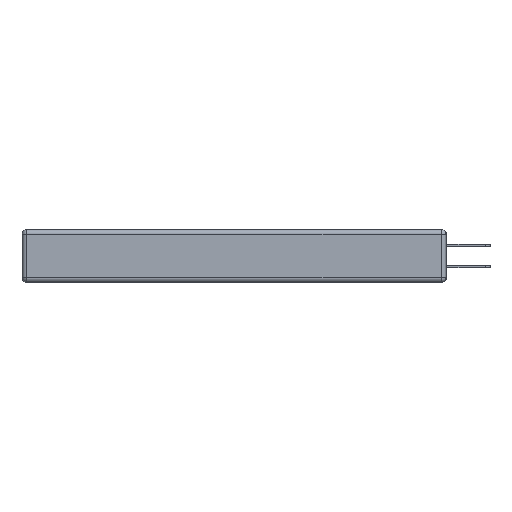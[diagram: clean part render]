
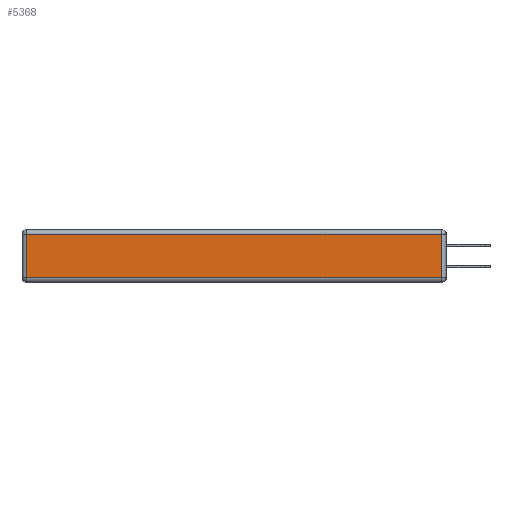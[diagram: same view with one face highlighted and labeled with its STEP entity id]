
A CAD part, left-side view. The second image highlights one B-rep face of the part: STEP entity #5368.
In plain terms, the highlighted planar face has unit normal (-1, 0, 0).
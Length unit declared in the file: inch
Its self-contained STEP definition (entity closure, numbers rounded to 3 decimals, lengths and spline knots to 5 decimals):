
#527 = VECTOR ( 'NONE', #2882, 39.37008 ) ;
#579 = EDGE_CURVE ( 'NONE', #10166, #8244, #9473, .T. ) ;
#781 = PLANE ( 'NONE',  #907 ) ;
#907 = AXIS2_PLACEMENT_3D ( 'NONE', #3985, #10316, #10239 ) ;
#2882 = DIRECTION ( 'NONE',  ( 0., 0., 1. ) ) ;
#3028 = CARTESIAN_POINT ( 'NONE',  ( 0., 2.72, -0.03 ) ) ;
#3032 = VECTOR ( 'NONE', #9479, 39.37008 ) ;
#3380 = ORIENTED_EDGE ( 'NONE', *, *, #13090, .T. ) ;
#3985 = CARTESIAN_POINT ( 'NONE',  ( 0., 0., -0.343 ) ) ;
#4539 = EDGE_CURVE ( 'NONE', #4904, #10166, #9600, .T. ) ;
#4622 = DIRECTION ( 'NONE',  ( 0., 0., -1. ) ) ;
#4904 = VERTEX_POINT ( 'NONE', #3028 ) ;
#5368 = ADVANCED_FACE ( 'NONE', ( #6109 ), #781, .T. ) ;
#5450 = CARTESIAN_POINT ( 'NONE',  ( 0., 0., -0.313 ) ) ;
#5457 = EDGE_CURVE ( 'NONE', #8244, #11411, #7799, .T. ) ;
#6109 = FACE_OUTER_BOUND ( 'NONE', #7015, .T. ) ;
#6338 = DIRECTION ( 'NONE',  ( 0., -1., 0. ) ) ;
#6563 = CARTESIAN_POINT ( 'NONE',  ( 0., 2.72, -0.313 ) ) ;
#7015 = EDGE_LOOP ( 'NONE', ( #10856, #9487, #3380, #12816 ) ) ;
#7376 = CARTESIAN_POINT ( 'NONE',  ( 0., 2.75, -0.03 ) ) ;
#7799 = LINE ( 'NONE', #8158, #527 ) ;
#7987 = VECTOR ( 'NONE', #4622, 39.37008 ) ;
#8158 = CARTESIAN_POINT ( 'NONE',  ( 0., 0.03, -0.343 ) ) ;
#8244 = VERTEX_POINT ( 'NONE', #8621 ) ;
#8621 = CARTESIAN_POINT ( 'NONE',  ( 0., 0.03, -0.313 ) ) ;
#8834 = CARTESIAN_POINT ( 'NONE',  ( 0., 2.72, -0.343 ) ) ;
#9473 = LINE ( 'NONE', #5450, #10459 ) ;
#9479 = DIRECTION ( 'NONE',  ( 0., 1., 0. ) ) ;
#9487 = ORIENTED_EDGE ( 'NONE', *, *, #5457, .T. ) ;
#9600 = LINE ( 'NONE', #8834, #7987 ) ;
#10166 = VERTEX_POINT ( 'NONE', #6563 ) ;
#10239 = DIRECTION ( 'NONE',  ( 0., 0., 1. ) ) ;
#10316 = DIRECTION ( 'NONE',  ( -1., 0., 0. ) ) ;
#10459 = VECTOR ( 'NONE', #6338, 39.37008 ) ;
#10811 = LINE ( 'NONE', #7376, #3032 ) ;
#10856 = ORIENTED_EDGE ( 'NONE', *, *, #579, .T. ) ;
#11411 = VERTEX_POINT ( 'NONE', #12409 ) ;
#12409 = CARTESIAN_POINT ( 'NONE',  ( 0., 0.03, -0.03 ) ) ;
#12816 = ORIENTED_EDGE ( 'NONE', *, *, #4539, .T. ) ;
#13090 = EDGE_CURVE ( 'NONE', #11411, #4904, #10811, .T. ) ;
